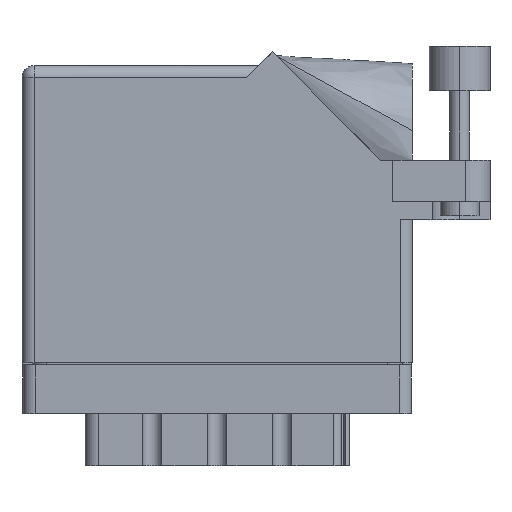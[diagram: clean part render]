
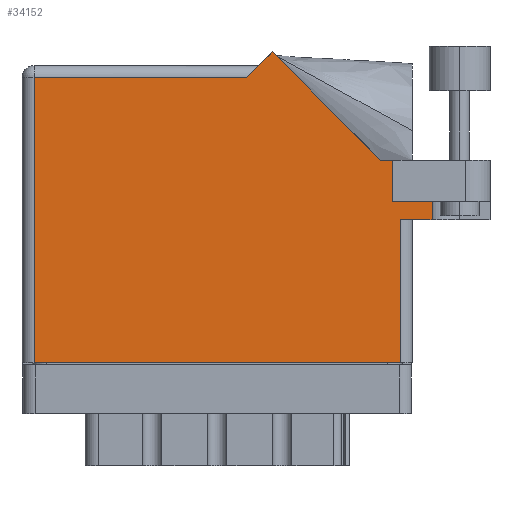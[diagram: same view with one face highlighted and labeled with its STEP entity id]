
A CAD part, front view. The second image highlights one B-rep face of the part: STEP entity #34152.
In plain terms, the highlighted face is planar.
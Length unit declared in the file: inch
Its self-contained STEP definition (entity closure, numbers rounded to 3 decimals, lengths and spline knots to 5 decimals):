
#224 = CARTESIAN_POINT ( 'NONE',  ( 1.84442, 1.044, 0. ) ) ;
#655 = DIRECTION ( 'NONE',  ( -1., 0., 0. ) ) ;
#776 = LINE ( 'NONE', #32182, #30784 ) ;
#1100 = ORIENTED_EDGE ( 'NONE', *, *, #33230, .T. ) ;
#1531 = VECTOR ( 'NONE', #20431, 39.37008 ) ;
#2578 = VERTEX_POINT ( 'NONE', #6351 ) ;
#2934 = CARTESIAN_POINT ( 'NONE',  ( 1.84442, 1.044, 0. ) ) ;
#3201 = CARTESIAN_POINT ( 'NONE',  ( 1.948, 0.737, 0. ) ) ;
#3435 = DIRECTION ( 'NONE',  ( -0.707, 0.707, 0. ) ) ;
#3572 = DIRECTION ( 'NONE',  ( 0., 1., 0. ) ) ;
#4068 = EDGE_CURVE ( 'NONE', #19460, #18182, #6400, .T. ) ;
#4556 = EDGE_CURVE ( 'NONE', #17855, #19460, #24137, .T. ) ;
#5296 = ORIENTED_EDGE ( 'NONE', *, *, #13256, .T. ) ;
#5473 = CARTESIAN_POINT ( 'NONE',  ( 1.91, 0.831, 0. ) ) ;
#5841 = EDGE_LOOP ( 'NONE', ( #20686, #35100, #5296, #32382, #36899, #1100, #34151, #17999, #12841, #32829, #36287 ) ) ;
#6290 = CARTESIAN_POINT ( 'NONE',  ( 1.948, 0.737, 0. ) ) ;
#6351 = CARTESIAN_POINT ( 'NONE',  ( 0.062, 0., 0. ) ) ;
#6400 = LINE ( 'NONE', #2934, #12757 ) ;
#6428 = EDGE_CURVE ( 'NONE', #24291, #2578, #37468, .T. ) ;
#6445 = CARTESIAN_POINT ( 'NONE',  ( 1.91, 0.831, 0. ) ) ;
#6780 = EDGE_CURVE ( 'NONE', #18182, #23253, #15642, .T. ) ;
#8009 = LINE ( 'NONE', #13354, #24392 ) ;
#8328 = AXIS2_PLACEMENT_3D ( 'NONE', #11644, #20463, #34814 ) ;
#8372 = CARTESIAN_POINT ( 'NONE',  ( 2.41, 1.044, 0. ) ) ;
#8755 = CARTESIAN_POINT ( 'NONE',  ( 2.1115, 1.16177, 0. ) ) ;
#8787 = DIRECTION ( 'NONE',  ( 1., 0., 0. ) ) ;
#11644 = CARTESIAN_POINT ( 'NONE',  ( 0., 1.53, 0. ) ) ;
#12757 = VECTOR ( 'NONE', #3435, 39.37008 ) ;
#12841 = ORIENTED_EDGE ( 'NONE', *, *, #6780, .T. ) ;
#13153 = VECTOR ( 'NONE', #17677, 39.37008 ) ;
#13256 = EDGE_CURVE ( 'NONE', #36909, #14426, #23671, .T. ) ;
#13354 = CARTESIAN_POINT ( 'NONE',  ( 1.91, 0.831, 0. ) ) ;
#13976 = VECTOR ( 'NONE', #32499, 39.37008 ) ;
#14135 = CARTESIAN_POINT ( 'NONE',  ( 2.1115, 0.737, 0. ) ) ;
#14426 = VERTEX_POINT ( 'NONE', #14135 ) ;
#14501 = CARTESIAN_POINT ( 'NONE',  ( 0., 1.468, 0. ) ) ;
#14706 = PLANE ( 'NONE',  #8328 ) ;
#15187 = FACE_OUTER_BOUND ( 'NONE', #5841, .T. ) ;
#15563 = EDGE_CURVE ( 'NONE', #2578, #33386, #776, .T. ) ;
#15642 = LINE ( 'NONE', #17868, #1531 ) ;
#15937 = VECTOR ( 'NONE', #21817, 39.37008 ) ;
#16392 = VECTOR ( 'NONE', #26169, 39.37008 ) ;
#17269 = CARTESIAN_POINT ( 'NONE',  ( 1.155, 1.468, 0. ) ) ;
#17677 = DIRECTION ( 'NONE',  ( 0., -1., 0. ) ) ;
#17855 = VERTEX_POINT ( 'NONE', #25230 ) ;
#17868 = CARTESIAN_POINT ( 'NONE',  ( 1.217, 1.53, 0. ) ) ;
#17999 = ORIENTED_EDGE ( 'NONE', *, *, #4068, .T. ) ;
#18182 = VERTEX_POINT ( 'NONE', #24307 ) ;
#18822 = DIRECTION ( 'NONE',  ( 0., -1., 0. ) ) ;
#19460 = VERTEX_POINT ( 'NONE', #224 ) ;
#20431 = DIRECTION ( 'NONE',  ( -0.707, -0.707, 0. ) ) ;
#20463 = DIRECTION ( 'NONE',  ( 0., 0., -1. ) ) ;
#20686 = ORIENTED_EDGE ( 'NONE', *, *, #15563, .T. ) ;
#21164 = VECTOR ( 'NONE', #655, 39.37008 ) ;
#21817 = DIRECTION ( 'NONE',  ( 1., 0., 0. ) ) ;
#22710 = EDGE_CURVE ( 'NONE', #28671, #14426, #33647, .T. ) ;
#23253 = VERTEX_POINT ( 'NONE', #17269 ) ;
#23671 = LINE ( 'NONE', #27549, #15937 ) ;
#24137 = LINE ( 'NONE', #8372, #16392 ) ;
#24291 = VERTEX_POINT ( 'NONE', #36984 ) ;
#24307 = CARTESIAN_POINT ( 'NONE',  ( 1.28771, 1.60071, 0. ) ) ;
#24392 = VECTOR ( 'NONE', #36366, 39.37008 ) ;
#25230 = CARTESIAN_POINT ( 'NONE',  ( 1.91, 1.044, 0. ) ) ;
#25588 = EDGE_CURVE ( 'NONE', #23253, #24291, #34808, .T. ) ;
#26169 = DIRECTION ( 'NONE',  ( -1., 0., 0. ) ) ;
#27549 = CARTESIAN_POINT ( 'NONE',  ( 2.01, 0.737, 0. ) ) ;
#27598 = CARTESIAN_POINT ( 'NONE',  ( 0.062, 0., 0. ) ) ;
#28183 = EDGE_CURVE ( 'NONE', #33386, #36909, #36423, .T. ) ;
#28263 = CARTESIAN_POINT ( 'NONE',  ( 1.948, 0., 0. ) ) ;
#28671 = VERTEX_POINT ( 'NONE', #36821 ) ;
#29780 = VECTOR ( 'NONE', #18822, 39.37008 ) ;
#30784 = VECTOR ( 'NONE', #8787, 39.37008 ) ;
#31474 = EDGE_CURVE ( 'NONE', #35624, #28671, #37636, .T. ) ;
#32182 = CARTESIAN_POINT ( 'NONE',  ( 0., 0., 0. ) ) ;
#32382 = ORIENTED_EDGE ( 'NONE', *, *, #22710, .F. ) ;
#32499 = DIRECTION ( 'NONE',  ( 1., 0., 0. ) ) ;
#32829 = ORIENTED_EDGE ( 'NONE', *, *, #25588, .T. ) ;
#33230 = EDGE_CURVE ( 'NONE', #35624, #17855, #8009, .T. ) ;
#33386 = VERTEX_POINT ( 'NONE', #28263 ) ;
#33647 = LINE ( 'NONE', #8755, #13153 ) ;
#34151 = ORIENTED_EDGE ( 'NONE', *, *, #4556, .T. ) ;
#34152 = ADVANCED_FACE ( 'NONE', ( #15187 ), #14706, .F. ) ;
#34808 = LINE ( 'NONE', #14501, #21164 ) ;
#34814 = DIRECTION ( 'NONE',  ( -1., 0., 0. ) ) ;
#35100 = ORIENTED_EDGE ( 'NONE', *, *, #28183, .T. ) ;
#35522 = VECTOR ( 'NONE', #3572, 39.37008 ) ;
#35624 = VERTEX_POINT ( 'NONE', #5473 ) ;
#36287 = ORIENTED_EDGE ( 'NONE', *, *, #6428, .T. ) ;
#36366 = DIRECTION ( 'NONE',  ( 0., 1., 0. ) ) ;
#36423 = LINE ( 'NONE', #3201, #35522 ) ;
#36821 = CARTESIAN_POINT ( 'NONE',  ( 2.1115, 0.831, 0. ) ) ;
#36899 = ORIENTED_EDGE ( 'NONE', *, *, #31474, .F. ) ;
#36909 = VERTEX_POINT ( 'NONE', #6290 ) ;
#36984 = CARTESIAN_POINT ( 'NONE',  ( 0.062, 1.468, 0. ) ) ;
#37468 = LINE ( 'NONE', #27598, #29780 ) ;
#37636 = LINE ( 'NONE', #6445, #13976 ) ;
